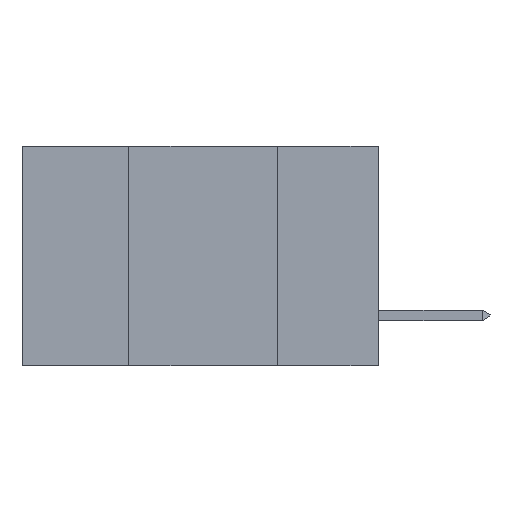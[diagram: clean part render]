
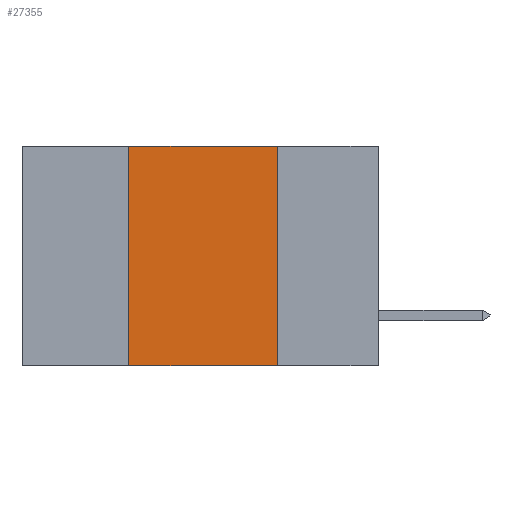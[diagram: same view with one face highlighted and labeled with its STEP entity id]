
A CAD part, left-side view. The second image highlights one B-rep face of the part: STEP entity #27355.
In plain terms, the highlighted planar face has unit normal (-1, 0, 0).
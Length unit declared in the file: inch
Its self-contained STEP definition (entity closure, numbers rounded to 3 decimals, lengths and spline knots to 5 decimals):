
#63 = VERTEX_POINT ( 'NONE', #5930 ) ;
#1606 = ORIENTED_EDGE ( 'NONE', *, *, #16558, .T. ) ;
#1733 = EDGE_CURVE ( 'NONE', #12434, #63, #23191, .T. ) ;
#3212 = CARTESIAN_POINT ( 'NONE',  ( 0., 0.42, -0.37 ) ) ;
#3369 = ORIENTED_EDGE ( 'NONE', *, *, #27139, .F. ) ;
#5591 = LINE ( 'NONE', #19576, #32398 ) ;
#5930 = CARTESIAN_POINT ( 'NONE',  ( 0., 0.17, -0.37 ) ) ;
#6888 = ORIENTED_EDGE ( 'NONE', *, *, #1733, .F. ) ;
#7818 = VERTEX_POINT ( 'NONE', #3212 ) ;
#10915 = LINE ( 'NONE', #20970, #30252 ) ;
#12181 = EDGE_LOOP ( 'NONE', ( #6888, #3369, #17685, #1606 ) ) ;
#12324 = DIRECTION ( 'NONE',  ( 0., 0., -1. ) ) ;
#12434 = VERTEX_POINT ( 'NONE', #22945 ) ;
#12556 = CARTESIAN_POINT ( 'NONE',  ( 0., 0.6, 0. ) ) ;
#13297 = VERTEX_POINT ( 'NONE', #28376 ) ;
#14990 = AXIS2_PLACEMENT_3D ( 'NONE', #12556, #24944, #29981 ) ;
#16057 = VECTOR ( 'NONE', #29905, 39.37008 ) ;
#16558 = EDGE_CURVE ( 'NONE', #7818, #63, #10915, .T. ) ;
#17685 = ORIENTED_EDGE ( 'NONE', *, *, #32403, .F. ) ;
#19576 = CARTESIAN_POINT ( 'NONE',  ( 0., 0.42, 0. ) ) ;
#19878 = PLANE ( 'NONE',  #14990 ) ;
#20970 = CARTESIAN_POINT ( 'NONE',  ( 0., 0.6, -0.37 ) ) ;
#22227 = CARTESIAN_POINT ( 'NONE',  ( 0., 0.6, 0. ) ) ;
#22945 = CARTESIAN_POINT ( 'NONE',  ( 0., 0.17, 0. ) ) ;
#23030 = DIRECTION ( 'NONE',  ( 0., -1., 0. ) ) ;
#23191 = LINE ( 'NONE', #24838, #25177 ) ;
#24838 = CARTESIAN_POINT ( 'NONE',  ( 0., 0.17, 0. ) ) ;
#24944 = DIRECTION ( 'NONE',  ( 1., 0., 0. ) ) ;
#25177 = VECTOR ( 'NONE', #12324, 39.37008 ) ;
#27139 = EDGE_CURVE ( 'NONE', #13297, #12434, #30283, .T. ) ;
#27355 = ADVANCED_FACE ( 'NONE', ( #28309 ), #19878, .F. ) ;
#28309 = FACE_OUTER_BOUND ( 'NONE', #12181, .T. ) ;
#28376 = CARTESIAN_POINT ( 'NONE',  ( 0., 0.42, 0. ) ) ;
#29905 = DIRECTION ( 'NONE',  ( 0., -1., 0. ) ) ;
#29981 = DIRECTION ( 'NONE',  ( 0., 0., -1. ) ) ;
#30252 = VECTOR ( 'NONE', #23030, 39.37008 ) ;
#30283 = LINE ( 'NONE', #22227, #16057 ) ;
#31996 = DIRECTION ( 'NONE',  ( 0., 0., 1. ) ) ;
#32398 = VECTOR ( 'NONE', #31996, 39.37008 ) ;
#32403 = EDGE_CURVE ( 'NONE', #7818, #13297, #5591, .T. ) ;
